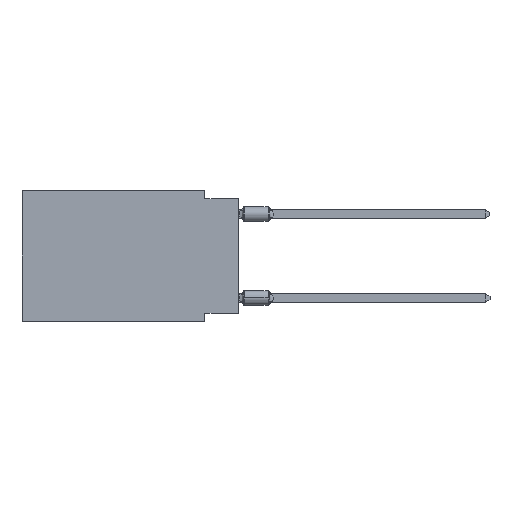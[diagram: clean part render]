
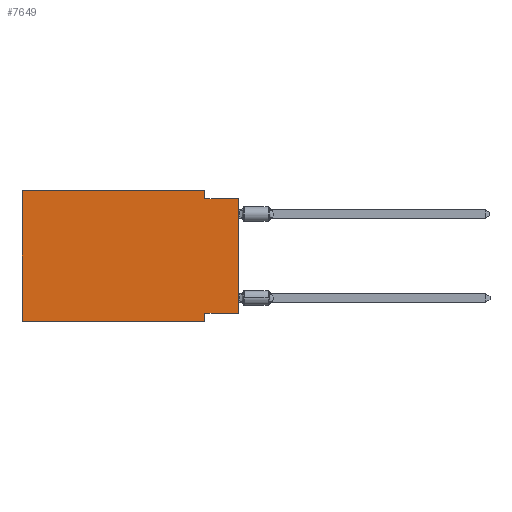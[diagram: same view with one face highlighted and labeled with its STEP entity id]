
A CAD part, left-side view. The second image highlights one B-rep face of the part: STEP entity #7649.
In plain terms, the highlighted planar face has unit normal (-1, 0, 0).
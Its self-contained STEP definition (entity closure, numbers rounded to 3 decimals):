
#1338 = ORIENTED_EDGE ( 'NONE', *, *, #13550, .T. ) ;
#1673 = CARTESIAN_POINT ( 'NONE',  ( 0., 2.54, 0. ) ) ;
#2084 = AXIS2_PLACEMENT_3D ( 'NONE', #19381, #3623, #11490 ) ;
#2249 = EDGE_CURVE ( 'NONE', #6101, #6001, #4946, .T. ) ;
#2549 = CARTESIAN_POINT ( 'NONE',  ( 0., 2.54, 0. ) ) ;
#3471 = DIRECTION ( 'NONE',  ( 0., 0., 1. ) ) ;
#3513 = VERTEX_POINT ( 'NONE', #7488 ) ;
#3623 = DIRECTION ( 'NONE',  ( 1., 0., 0. ) ) ;
#3665 = ORIENTED_EDGE ( 'NONE', *, *, #18327, .F. ) ;
#4348 = VECTOR ( 'NONE', #15344, 1000. ) ;
#4362 = LINE ( 'NONE', #2549, #23322 ) ;
#4407 = EDGE_CURVE ( 'NONE', #24858, #23184, #4362, .T. ) ;
#4440 = VECTOR ( 'NONE', #7903, 1000. ) ;
#4946 = LINE ( 'NONE', #6497, #23915 ) ;
#5213 = EDGE_LOOP ( 'NONE', ( #1338, #24697, #5859, #6090, #20386, #17277, #3665, #11273 ) ) ;
#5442 = VECTOR ( 'NONE', #6071, 1000. ) ;
#5859 = ORIENTED_EDGE ( 'NONE', *, *, #4407, .F. ) ;
#6001 = VERTEX_POINT ( 'NONE', #9883 ) ;
#6071 = DIRECTION ( 'NONE',  ( 0., -1., 0. ) ) ;
#6090 = ORIENTED_EDGE ( 'NONE', *, *, #16761, .F. ) ;
#6101 = VERTEX_POINT ( 'NONE', #12340 ) ;
#6125 = LINE ( 'NONE', #24218, #21469 ) ;
#6497 = CARTESIAN_POINT ( 'NONE',  ( 0., 16.383, -9.906 ) ) ;
#7488 = CARTESIAN_POINT ( 'NONE',  ( 0., 2.54, -9.271 ) ) ;
#7649 = ADVANCED_FACE ( 'NONE', ( #17302 ), #21319, .F. ) ;
#7903 = DIRECTION ( 'NONE',  ( 0., -1., 0. ) ) ;
#7936 = CARTESIAN_POINT ( 'NONE',  ( 0., 0., -9.271 ) ) ;
#8548 = DIRECTION ( 'NONE',  ( 0., -1., 0. ) ) ;
#9883 = CARTESIAN_POINT ( 'NONE',  ( 0., 2.54, -9.906 ) ) ;
#9938 = CARTESIAN_POINT ( 'NONE',  ( 0., 16.383, 0. ) ) ;
#10064 = CARTESIAN_POINT ( 'NONE',  ( 0., 0., -0.635 ) ) ;
#10772 = VECTOR ( 'NONE', #3471, 1000. ) ;
#11273 = ORIENTED_EDGE ( 'NONE', *, *, #17412, .F. ) ;
#11344 = VERTEX_POINT ( 'NONE', #15493 ) ;
#11490 = DIRECTION ( 'NONE',  ( 0., 0., -1. ) ) ;
#11601 = LINE ( 'NONE', #22040, #10772 ) ;
#11886 = CARTESIAN_POINT ( 'NONE',  ( 0., 2.54, -9.906 ) ) ;
#12340 = CARTESIAN_POINT ( 'NONE',  ( 0., 16.383, -9.906 ) ) ;
#13550 = EDGE_CURVE ( 'NONE', #22166, #11344, #6125, .T. ) ;
#13819 = LINE ( 'NONE', #11886, #24590 ) ;
#14192 = EDGE_CURVE ( 'NONE', #6101, #14288, #11601, .T. ) ;
#14288 = VERTEX_POINT ( 'NONE', #9938 ) ;
#14850 = LINE ( 'NONE', #22850, #4348 ) ;
#15344 = DIRECTION ( 'NONE',  ( 0., 1., 0. ) ) ;
#15493 = CARTESIAN_POINT ( 'NONE',  ( 0., 0., -0.635 ) ) ;
#15529 = EDGE_CURVE ( 'NONE', #23184, #11344, #18073, .T. ) ;
#16761 = EDGE_CURVE ( 'NONE', #14288, #24858, #17587, .T. ) ;
#17277 = ORIENTED_EDGE ( 'NONE', *, *, #2249, .T. ) ;
#17302 = FACE_OUTER_BOUND ( 'NONE', #5213, .T. ) ;
#17412 = EDGE_CURVE ( 'NONE', #22166, #3513, #14850, .T. ) ;
#17587 = LINE ( 'NONE', #21737, #4440 ) ;
#18073 = LINE ( 'NONE', #10064, #5442 ) ;
#18327 = EDGE_CURVE ( 'NONE', #3513, #6001, #13819, .T. ) ;
#18381 = DIRECTION ( 'NONE',  ( 0., 0., 1. ) ) ;
#19381 = CARTESIAN_POINT ( 'NONE',  ( 0., 16.383, 0. ) ) ;
#20030 = CARTESIAN_POINT ( 'NONE',  ( 0., 2.54, -0.635 ) ) ;
#20386 = ORIENTED_EDGE ( 'NONE', *, *, #14192, .F. ) ;
#21319 = PLANE ( 'NONE',  #2084 ) ;
#21469 = VECTOR ( 'NONE', #18381, 1000. ) ;
#21710 = DIRECTION ( 'NONE',  ( 0., 0., -1. ) ) ;
#21737 = CARTESIAN_POINT ( 'NONE',  ( 0., 16.383, 0. ) ) ;
#21804 = DIRECTION ( 'NONE',  ( 0., 0., -1. ) ) ;
#22040 = CARTESIAN_POINT ( 'NONE',  ( 0., 16.383, 0. ) ) ;
#22166 = VERTEX_POINT ( 'NONE', #7936 ) ;
#22850 = CARTESIAN_POINT ( 'NONE',  ( 0., 0., -9.271 ) ) ;
#23184 = VERTEX_POINT ( 'NONE', #20030 ) ;
#23322 = VECTOR ( 'NONE', #21804, 1000. ) ;
#23915 = VECTOR ( 'NONE', #8548, 1000. ) ;
#24218 = CARTESIAN_POINT ( 'NONE',  ( 0., 0., 0. ) ) ;
#24590 = VECTOR ( 'NONE', #21710, 1000. ) ;
#24697 = ORIENTED_EDGE ( 'NONE', *, *, #15529, .F. ) ;
#24858 = VERTEX_POINT ( 'NONE', #1673 ) ;
